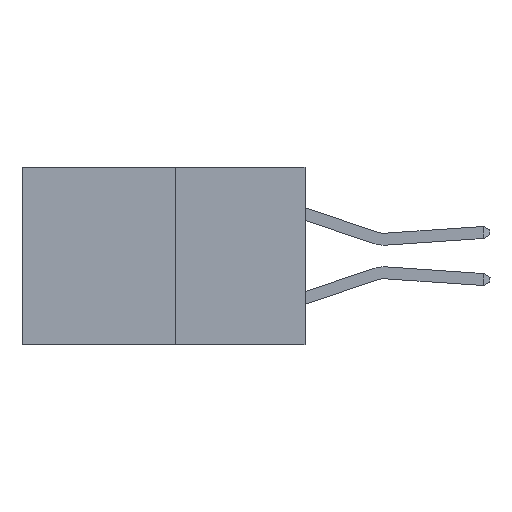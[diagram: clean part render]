
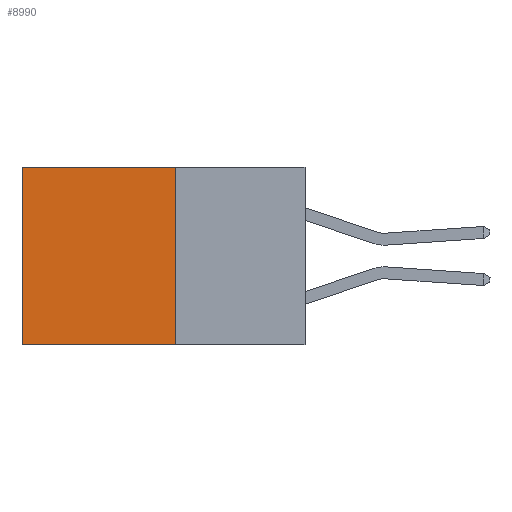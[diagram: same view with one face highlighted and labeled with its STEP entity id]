
A CAD part, left-side view. The second image highlights one B-rep face of the part: STEP entity #8990.
In plain terms, the highlighted planar face has unit normal (-1, 0, 0).
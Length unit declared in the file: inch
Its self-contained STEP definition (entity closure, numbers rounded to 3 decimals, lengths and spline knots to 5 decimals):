
#649 = FACE_OUTER_BOUND ( 'NONE', #16014, .T. ) ;
#1155 = VERTEX_POINT ( 'NONE', #3309 ) ;
#1643 = VERTEX_POINT ( 'NONE', #9935 ) ;
#1943 = DIRECTION ( 'NONE',  ( 0., 0., -1. ) ) ;
#2014 = VECTOR ( 'NONE', #2564, 39.37008 ) ;
#2048 = LINE ( 'NONE', #10188, #5973 ) ;
#2564 = DIRECTION ( 'NONE',  ( 0., 0., -1. ) ) ;
#2642 = VECTOR ( 'NONE', #10565, 39.37008 ) ;
#2881 = AXIS2_PLACEMENT_3D ( 'NONE', #8120, #7870, #7842 ) ;
#3309 = CARTESIAN_POINT ( 'NONE',  ( 0.277, 0.59, 0. ) ) ;
#3549 = LINE ( 'NONE', #12758, #15990 ) ;
#3696 = LINE ( 'NONE', #10901, #2642 ) ;
#5973 = VECTOR ( 'NONE', #1943, 39.37008 ) ;
#6418 = EDGE_CURVE ( 'NONE', #16689, #1643, #3696, .T. ) ;
#7842 = DIRECTION ( 'NONE',  ( 0., 0., -1. ) ) ;
#7870 = DIRECTION ( 'NONE',  ( 1., 0., 0. ) ) ;
#7938 = PLANE ( 'NONE',  #2881 ) ;
#8120 = CARTESIAN_POINT ( 'NONE',  ( 0.277, 0.27, -0.37 ) ) ;
#8704 = ORIENTED_EDGE ( 'NONE', *, *, #10463, .T. ) ;
#8959 = CARTESIAN_POINT ( 'NONE',  ( 0.277, 0.27, -0.37 ) ) ;
#8990 = ADVANCED_FACE ( 'NONE', ( #649 ), #7938, .F. ) ;
#9141 = CARTESIAN_POINT ( 'NONE',  ( 0.277, 0.59, -0.37 ) ) ;
#9935 = CARTESIAN_POINT ( 'NONE',  ( 0.277, 0.59, -0.37 ) ) ;
#10188 = CARTESIAN_POINT ( 'NONE',  ( 0.277, 0.27, -0.37 ) ) ;
#10463 = EDGE_CURVE ( 'NONE', #12026, #1155, #3549, .T. ) ;
#10565 = DIRECTION ( 'NONE',  ( 0., 1., 0. ) ) ;
#10901 = CARTESIAN_POINT ( 'NONE',  ( 0.277, 0.27, -0.37 ) ) ;
#12026 = VERTEX_POINT ( 'NONE', #14712 ) ;
#12319 = ORIENTED_EDGE ( 'NONE', *, *, #6418, .F. ) ;
#12485 = ORIENTED_EDGE ( 'NONE', *, *, #15902, .T. ) ;
#12758 = CARTESIAN_POINT ( 'NONE',  ( 0.277, 0.27, 0. ) ) ;
#14712 = CARTESIAN_POINT ( 'NONE',  ( 0.277, 0.27, 0. ) ) ;
#15076 = EDGE_CURVE ( 'NONE', #12026, #16689, #2048, .T. ) ;
#15902 = EDGE_CURVE ( 'NONE', #1155, #1643, #19220, .T. ) ;
#15916 = DIRECTION ( 'NONE',  ( 0., 1., 0. ) ) ;
#15990 = VECTOR ( 'NONE', #15916, 39.37008 ) ;
#16014 = EDGE_LOOP ( 'NONE', ( #12485, #12319, #20278, #8704 ) ) ;
#16689 = VERTEX_POINT ( 'NONE', #8959 ) ;
#19220 = LINE ( 'NONE', #9141, #2014 ) ;
#20278 = ORIENTED_EDGE ( 'NONE', *, *, #15076, .F. ) ;
